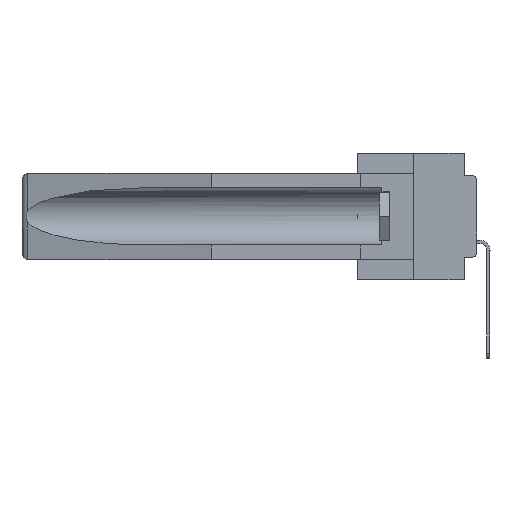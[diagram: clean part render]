
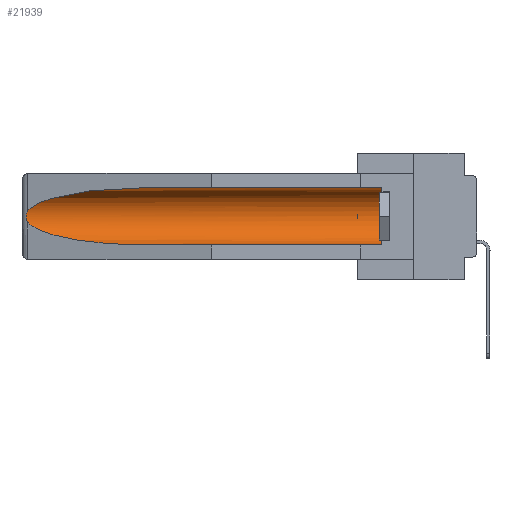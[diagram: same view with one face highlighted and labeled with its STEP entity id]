
A CAD part, left-side view. The second image highlights one B-rep face of the part: STEP entity #21939.
In plain terms, the highlighted cylindrical face has radius 2.857 mm (diameter 5.715 mm), a partial arc.
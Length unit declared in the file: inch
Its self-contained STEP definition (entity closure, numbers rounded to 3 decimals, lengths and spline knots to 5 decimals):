
#280 = CARTESIAN_POINT ( 'NONE',  ( 0.155, -0.30754, -0.284 ) ) ;
#1282 = LINE ( 'NONE', #35517, #20647 ) ;
#1730 = CARTESIAN_POINT ( 'NONE',  ( 0.26597, 1.5296, -0.19026 ) ) ;
#2319 =( BOUNDED_CURVE ( )  B_SPLINE_CURVE ( 3, ( #8994, #36941, #24171, #14689 ),
 .UNSPECIFIED., .F., .F. ) 
 B_SPLINE_CURVE_WITH_KNOTS ( ( 4, 4 ),
 ( 0.1948, 1.5708 ),
 .UNSPECIFIED. ) 
 CURVE ( )  GEOMETRIC_REPRESENTATION_ITEM ( )  RATIONAL_B_SPLINE_CURVE ( ( 1., 0.848, 0.848, 1. ) ) 
 REPRESENTATION_ITEM ( '' )  );
#2805 = DIRECTION ( 'NONE',  ( 0., -1., 0. ) ) ;
#3244 = AXIS2_PLACEMENT_3D ( 'NONE', #24264, #2805, #5844 ) ;
#3614 = CARTESIAN_POINT ( 'NONE',  ( 0.21114, 1.30732, -0.059 ) ) ;
#4362 = CARTESIAN_POINT ( 'NONE',  ( 0.26537, 1.52718, -0.14972 ) ) ;
#4972 = CARTESIAN_POINT ( 'NONE',  ( 0.26537, 1.52718, -0.19328 ) ) ;
#5844 = DIRECTION ( 'NONE',  ( 0., 0., 1. ) ) ;
#6353 = DIRECTION ( 'NONE',  ( 0., 1., 0. ) ) ;
#7422 = CARTESIAN_POINT ( 'NONE',  ( 0.26597, 1.52961, -0.15275 ) ) ;
#7616 = CARTESIAN_POINT ( 'NONE',  ( 0.2675, 1.53308, -0.17534 ) ) ;
#7764 = DIRECTION ( 'NONE',  ( 0., 1., 0. ) ) ;
#7814 = CARTESIAN_POINT ( 'NONE',  ( 0.2673, 1.5327, -0.16383 ) ) ;
#7973 = DIRECTION ( 'NONE',  ( 0., 0., 1. ) ) ;
#8022 = CARTESIAN_POINT ( 'NONE',  ( 0.2675, 1.53308, -0.16763 ) ) ;
#8994 = CARTESIAN_POINT ( 'NONE',  ( 0.26537, 1.52718, -0.19328 ) ) ;
#9292 =( BOUNDED_CURVE ( )  B_SPLINE_CURVE ( 3, ( #21639, #3614, #31173, #9698 ),
 .UNSPECIFIED., .F., .F. ) 
 B_SPLINE_CURVE_WITH_KNOTS ( ( 4, 4 ),
 ( 4.71239, 6.08839 ),
 .UNSPECIFIED. ) 
 CURVE ( )  GEOMETRIC_REPRESENTATION_ITEM ( )  RATIONAL_B_SPLINE_CURVE ( ( 1., 0.848, 0.848, 1. ) ) 
 REPRESENTATION_ITEM ( '' )  );
#9503 = EDGE_CURVE ( 'NONE', #39443, #33139, #2319, .T. ) ;
#9698 = CARTESIAN_POINT ( 'NONE',  ( 0.26537, 1.52718, -0.14972 ) ) ;
#9710 = CARTESIAN_POINT ( 'NONE',  ( 0.155, 0.126, -0.284 ) ) ;
#11169 = ORIENTED_EDGE ( 'NONE', *, *, #23941, .T. ) ;
#11206 = VERTEX_POINT ( 'NONE', #24416 ) ;
#12855 = ORIENTED_EDGE ( 'NONE', *, *, #15543, .T. ) ;
#14449 = VECTOR ( 'NONE', #6353, 39.37008 ) ;
#14689 = CARTESIAN_POINT ( 'NONE',  ( 0.155, 1.07973, -0.284 ) ) ;
#15053 = ORIENTED_EDGE ( 'NONE', *, *, #30456, .T. ) ;
#15179 = ORIENTED_EDGE ( 'NONE', *, *, #35346, .F. ) ;
#15543 = EDGE_CURVE ( 'NONE', #39048, #36272, #9292, .T. ) ;
#16690 = FACE_OUTER_BOUND ( 'NONE', #25556, .T. ) ;
#20369 = CARTESIAN_POINT ( 'NONE',  ( 0.26655, 1.53094, -0.18657 ) ) ;
#20450 = CARTESIAN_POINT ( 'NONE',  ( 0.26537, 1.52718, -0.19328 ) ) ;
#20647 = VECTOR ( 'NONE', #7764, 39.37008 ) ;
#21639 = CARTESIAN_POINT ( 'NONE',  ( 0.155, 1.07973, -0.059 ) ) ;
#21939 = ADVANCED_FACE ( 'NONE', ( #16690 ), #26408, .F. ) ;
#23941 = EDGE_CURVE ( 'NONE', #36272, #39443, #32478, .T. ) ;
#24171 = CARTESIAN_POINT ( 'NONE',  ( 0.21114, 1.30732, -0.284 ) ) ;
#24264 = CARTESIAN_POINT ( 'NONE',  ( 0.155, 0.126, -0.1715 ) ) ;
#24416 = CARTESIAN_POINT ( 'NONE',  ( 0.155, 0.126, -0.059 ) ) ;
#25366 = CARTESIAN_POINT ( 'NONE',  ( 0.155, 1.07973, -0.284 ) ) ;
#25556 = EDGE_LOOP ( 'NONE', ( #12855, #11169, #38070, #15179, #29958, #15053 ) ) ;
#25642 = CARTESIAN_POINT ( 'NONE',  ( 0.26537, 1.52718, -0.14972 ) ) ;
#26001 = CARTESIAN_POINT ( 'NONE',  ( 0.155, -0.30754, -0.1715 ) ) ;
#26408 = CYLINDRICAL_SURFACE ( 'NONE', #28700, 0.1125 ) ;
#26714 = CARTESIAN_POINT ( 'NONE',  ( 0.155, 1.07973, -0.059 ) ) ;
#28227 = LINE ( 'NONE', #280, #14449 ) ;
#28700 = AXIS2_PLACEMENT_3D ( 'NONE', #26001, #32285, #7973 ) ;
#29958 = ORIENTED_EDGE ( 'NONE', *, *, #32613, .T. ) ;
#30456 = EDGE_CURVE ( 'NONE', #11206, #39048, #1282, .T. ) ;
#30694 = VERTEX_POINT ( 'NONE', #9710 ) ;
#31173 = CARTESIAN_POINT ( 'NONE',  ( 0.25451, 1.48313, -0.09465 ) ) ;
#32285 = DIRECTION ( 'NONE',  ( 0., 1., 0. ) ) ;
#32478 = B_SPLINE_CURVE_WITH_KNOTS ( 'NONE', 3,
 ( #4362, #7422, #35767, #7814, #8022, #7616, #38399, #20369, #1730, #4972 ),
 .UNSPECIFIED., .F., .F.,
 ( 4, 2, 2, 2, 4 ),
 ( 0., 0.00029, 0.00058, 0.00087, 0.00117 ),
 .UNSPECIFIED. ) ;
#32613 = EDGE_CURVE ( 'NONE', #30694, #11206, #39459, .T. ) ;
#33139 = VERTEX_POINT ( 'NONE', #25366 ) ;
#35346 = EDGE_CURVE ( 'NONE', #30694, #33139, #28227, .T. ) ;
#35517 = CARTESIAN_POINT ( 'NONE',  ( 0.155, -0.30754, -0.059 ) ) ;
#35767 = CARTESIAN_POINT ( 'NONE',  ( 0.26654, 1.53092, -0.15636 ) ) ;
#36272 = VERTEX_POINT ( 'NONE', #25642 ) ;
#36941 = CARTESIAN_POINT ( 'NONE',  ( 0.25451, 1.48313, -0.24835 ) ) ;
#38070 = ORIENTED_EDGE ( 'NONE', *, *, #9503, .T. ) ;
#38399 = CARTESIAN_POINT ( 'NONE',  ( 0.2673, 1.53269, -0.17917 ) ) ;
#39048 = VERTEX_POINT ( 'NONE', #26714 ) ;
#39443 = VERTEX_POINT ( 'NONE', #20450 ) ;
#39459 = CIRCLE ( 'NONE', #3244, 0.1125 ) ;
